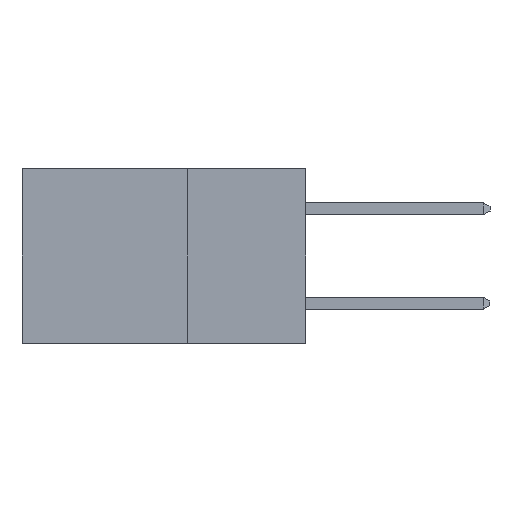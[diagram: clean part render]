
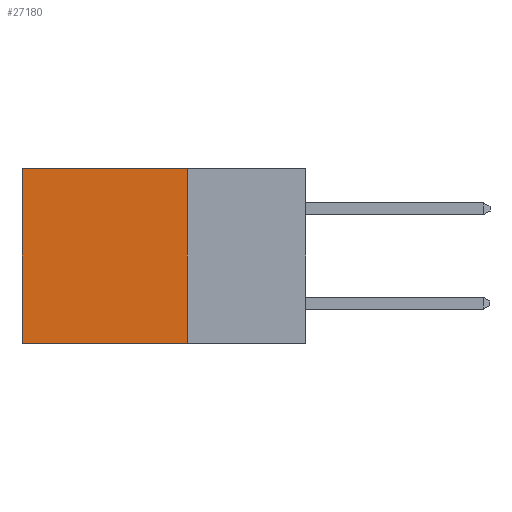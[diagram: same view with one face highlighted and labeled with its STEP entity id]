
A CAD part, left-side view. The second image highlights one B-rep face of the part: STEP entity #27180.
In plain terms, the highlighted planar face has unit normal (-1, 0, 0).
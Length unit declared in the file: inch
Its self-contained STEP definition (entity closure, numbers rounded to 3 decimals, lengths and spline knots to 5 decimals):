
#764 = VECTOR ( 'NONE', #15576, 39.37008 ) ;
#1180 = ORIENTED_EDGE ( 'NONE', *, *, #18841, .F. ) ;
#2789 = ORIENTED_EDGE ( 'NONE', *, *, #28428, .T. ) ;
#3241 = VECTOR ( 'NONE', #21401, 39.37008 ) ;
#3717 = CARTESIAN_POINT ( 'NONE',  ( 0.298, 0.6, 0. ) ) ;
#4084 = CARTESIAN_POINT ( 'NONE',  ( 0.298, 0.25, 0. ) ) ;
#5133 = CARTESIAN_POINT ( 'NONE',  ( 0.298, 0.6, 0. ) ) ;
#6830 = LINE ( 'NONE', #22076, #764 ) ;
#8520 = VECTOR ( 'NONE', #23604, 39.37008 ) ;
#8658 = DIRECTION ( 'NONE',  ( 0., 0., -1. ) ) ;
#8704 = EDGE_LOOP ( 'NONE', ( #2789, #1180, #13226, #9984 ) ) ;
#9103 = AXIS2_PLACEMENT_3D ( 'NONE', #4084, #21771, #8658 ) ;
#9984 = ORIENTED_EDGE ( 'NONE', *, *, #17142, .T. ) ;
#12597 = CARTESIAN_POINT ( 'NONE',  ( 0.298, 0.6, -0.37 ) ) ;
#13226 = ORIENTED_EDGE ( 'NONE', *, *, #21528, .F. ) ;
#15120 = LINE ( 'NONE', #19184, #3241 ) ;
#15300 = CARTESIAN_POINT ( 'NONE',  ( 0.298, 0.25, -0.37 ) ) ;
#15567 = LINE ( 'NONE', #19223, #26438 ) ;
#15576 = DIRECTION ( 'NONE',  ( 0., 1., 0. ) ) ;
#16618 = VERTEX_POINT ( 'NONE', #5133 ) ;
#17027 = VERTEX_POINT ( 'NONE', #15300 ) ;
#17142 = EDGE_CURVE ( 'NONE', #18135, #16618, #6830, .T. ) ;
#18135 = VERTEX_POINT ( 'NONE', #25343 ) ;
#18841 = EDGE_CURVE ( 'NONE', #17027, #19394, #15567, .T. ) ;
#19184 = CARTESIAN_POINT ( 'NONE',  ( 0.298, 0.25, 0. ) ) ;
#19223 = CARTESIAN_POINT ( 'NONE',  ( 0.298, 0.25, -0.37 ) ) ;
#19394 = VERTEX_POINT ( 'NONE', #12597 ) ;
#21401 = DIRECTION ( 'NONE',  ( 0., 0., -1. ) ) ;
#21431 = DIRECTION ( 'NONE',  ( 0., 1., 0. ) ) ;
#21528 = EDGE_CURVE ( 'NONE', #18135, #17027, #15120, .T. ) ;
#21771 = DIRECTION ( 'NONE',  ( 1., 0., 0. ) ) ;
#22076 = CARTESIAN_POINT ( 'NONE',  ( 0.298, 0.25, 0. ) ) ;
#23604 = DIRECTION ( 'NONE',  ( 0., 0., -1. ) ) ;
#23994 = FACE_OUTER_BOUND ( 'NONE', #8704, .T. ) ;
#25343 = CARTESIAN_POINT ( 'NONE',  ( 0.298, 0.25, 0. ) ) ;
#25938 = LINE ( 'NONE', #3717, #8520 ) ;
#26438 = VECTOR ( 'NONE', #21431, 39.37008 ) ;
#27180 = ADVANCED_FACE ( 'NONE', ( #23994 ), #28178, .F. ) ;
#28178 = PLANE ( 'NONE',  #9103 ) ;
#28428 = EDGE_CURVE ( 'NONE', #16618, #19394, #25938, .T. ) ;
